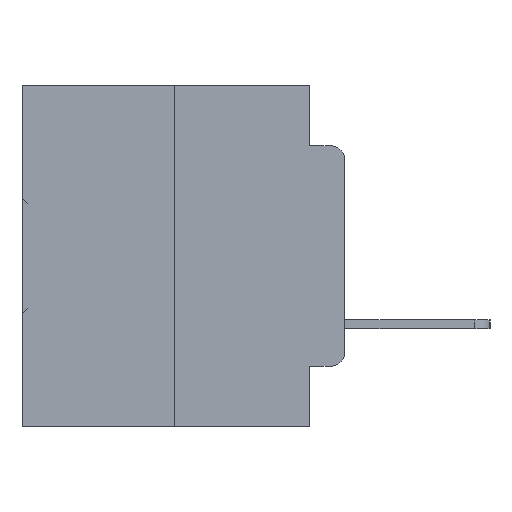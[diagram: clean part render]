
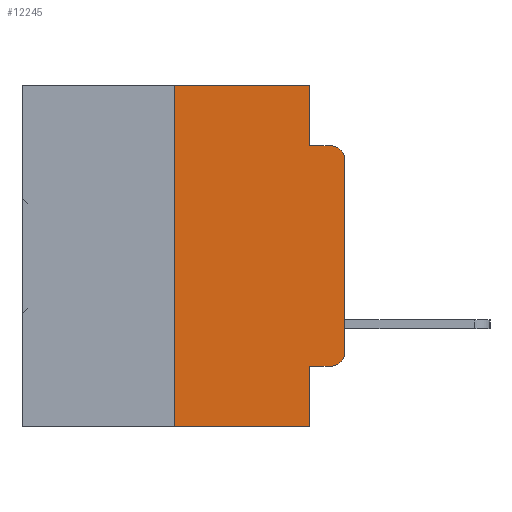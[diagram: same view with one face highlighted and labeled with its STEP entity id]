
A CAD part, left-side view. The second image highlights one B-rep face of the part: STEP entity #12245.
In plain terms, the highlighted planar face has unit normal (-1, 0, 0).
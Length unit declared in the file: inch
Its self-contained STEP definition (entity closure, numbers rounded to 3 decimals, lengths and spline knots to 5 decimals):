
#124 = ORIENTED_EDGE ( 'NONE', *, *, #3405, .T. ) ;
#536 = ORIENTED_EDGE ( 'NONE', *, *, #18207, .F. ) ;
#1031 = CARTESIAN_POINT ( 'NONE',  ( 0., 0.473, -0.5 ) ) ;
#1836 = DIRECTION ( 'NONE',  ( 0., -1., 0. ) ) ;
#2070 = VERTEX_POINT ( 'NONE', #21297 ) ;
#2082 = VERTEX_POINT ( 'NONE', #9404 ) ;
#2098 = CARTESIAN_POINT ( 'NONE',  ( 0., 0.051, -0.0885 ) ) ;
#3405 = EDGE_CURVE ( 'NONE', #30438, #2070, #6796, .T. ) ;
#4148 = DIRECTION ( 'NONE',  ( -1., 0., 0. ) ) ;
#4160 = CARTESIAN_POINT ( 'NONE',  ( 0., 0.051, 0. ) ) ;
#4267 = DIRECTION ( 'NONE',  ( 1., 0., 0. ) ) ;
#4569 = VECTOR ( 'NONE', #27969, 39.37008 ) ;
#4851 = DIRECTION ( 'NONE',  ( 0., -1., 0. ) ) ;
#5417 = LINE ( 'NONE', #4160, #4569 ) ;
#5450 = EDGE_CURVE ( 'NONE', #16482, #11013, #6231, .T. ) ;
#5864 = CARTESIAN_POINT ( 'NONE',  ( 0., 0.25, -0.5 ) ) ;
#5996 = VECTOR ( 'NONE', #30083, 39.37008 ) ;
#6231 = LINE ( 'NONE', #1031, #26460 ) ;
#6551 = DIRECTION ( 'NONE',  ( 0., -1., 0. ) ) ;
#6796 = CIRCLE ( 'NONE', #13078, 0.02 ) ;
#7189 = VERTEX_POINT ( 'NONE', #29967 ) ;
#7971 = EDGE_CURVE ( 'NONE', #2070, #7189, #33920, .T. ) ;
#8220 = CARTESIAN_POINT ( 'NONE',  ( 0., 0.051, -0.5 ) ) ;
#8527 = VECTOR ( 'NONE', #4851, 39.37008 ) ;
#9050 = LINE ( 'NONE', #16271, #15274 ) ;
#9404 = CARTESIAN_POINT ( 'NONE',  ( 0., 0.051, -0.4115 ) ) ;
#9470 = DIRECTION ( 'NONE',  ( -1., 0., 0. ) ) ;
#9798 = EDGE_CURVE ( 'NONE', #7189, #18177, #15871, .T. ) ;
#10254 = VERTEX_POINT ( 'NONE', #13930 ) ;
#11013 = VERTEX_POINT ( 'NONE', #8220 ) ;
#11117 = DIRECTION ( 'NONE',  ( 0., 0., -1. ) ) ;
#12245 = ADVANCED_FACE ( 'NONE', ( #18912 ), #17545, .F. ) ;
#12607 = CARTESIAN_POINT ( 'NONE',  ( 0., 0.051, -0.4115 ) ) ;
#12986 = DIRECTION ( 'NONE',  ( 0., -1., 0. ) ) ;
#13078 = AXIS2_PLACEMENT_3D ( 'NONE', #20061, #4148, #22706 ) ;
#13301 = VECTOR ( 'NONE', #1836, 39.37008 ) ;
#13930 = CARTESIAN_POINT ( 'NONE',  ( 0., 0.25, 0. ) ) ;
#14205 = EDGE_CURVE ( 'NONE', #2082, #30438, #34052, .T. ) ;
#14231 = CARTESIAN_POINT ( 'NONE',  ( 0., 0.051, 0. ) ) ;
#14738 = LINE ( 'NONE', #18208, #20865 ) ;
#14857 = CARTESIAN_POINT ( 'NONE',  ( 0., 0.02, -0.4115 ) ) ;
#15274 = VECTOR ( 'NONE', #11117, 39.37008 ) ;
#15871 = CIRCLE ( 'NONE', #29210, 0.02 ) ;
#15982 = EDGE_CURVE ( 'NONE', #2082, #11013, #9050, .T. ) ;
#16271 = CARTESIAN_POINT ( 'NONE',  ( 0., 0.051, 0. ) ) ;
#16482 = VERTEX_POINT ( 'NONE', #5864 ) ;
#17545 = PLANE ( 'NONE',  #25097 ) ;
#18161 = EDGE_CURVE ( 'NONE', #31803, #18177, #29434, .T. ) ;
#18177 = VERTEX_POINT ( 'NONE', #20736 ) ;
#18207 = EDGE_CURVE ( 'NONE', #10254, #21811, #14738, .T. ) ;
#18208 = CARTESIAN_POINT ( 'NONE',  ( 0., 0.473, 0. ) ) ;
#18912 = FACE_OUTER_BOUND ( 'NONE', #21444, .T. ) ;
#19676 = VECTOR ( 'NONE', #30300, 39.37008 ) ;
#20061 = CARTESIAN_POINT ( 'NONE',  ( 0., 0.02, -0.3915 ) ) ;
#20204 = ORIENTED_EDGE ( 'NONE', *, *, #18161, .F. ) ;
#20512 = LINE ( 'NONE', #22442, #19676 ) ;
#20582 = EDGE_CURVE ( 'NONE', #21811, #31803, #5417, .T. ) ;
#20736 = CARTESIAN_POINT ( 'NONE',  ( 0., 0.02, -0.0885 ) ) ;
#20865 = VECTOR ( 'NONE', #12986, 39.37008 ) ;
#21297 = CARTESIAN_POINT ( 'NONE',  ( 0., 0., -0.3915 ) ) ;
#21444 = EDGE_LOOP ( 'NONE', ( #31603, #32397, #20204, #34029, #536, #29586, #23498, #25140, #33646, #124 ) ) ;
#21642 = CARTESIAN_POINT ( 'NONE',  ( 0., 0.051, -0.0885 ) ) ;
#21811 = VERTEX_POINT ( 'NONE', #14231 ) ;
#22235 = CARTESIAN_POINT ( 'NONE',  ( 0., 0., 0. ) ) ;
#22442 = CARTESIAN_POINT ( 'NONE',  ( 0., 0.25, 0. ) ) ;
#22706 = DIRECTION ( 'NONE',  ( 0., 0., -1. ) ) ;
#22707 = CARTESIAN_POINT ( 'NONE',  ( 0., 0.473, 0. ) ) ;
#22818 = DIRECTION ( 'NONE',  ( 0., 0., -1. ) ) ;
#23498 = ORIENTED_EDGE ( 'NONE', *, *, #5450, .T. ) ;
#25097 = AXIS2_PLACEMENT_3D ( 'NONE', #22707, #4267, #22818 ) ;
#25140 = ORIENTED_EDGE ( 'NONE', *, *, #15982, .F. ) ;
#25181 = CARTESIAN_POINT ( 'NONE',  ( 0., 0.02, -0.1085 ) ) ;
#26460 = VECTOR ( 'NONE', #6551, 39.37008 ) ;
#27777 = DIRECTION ( 'NONE',  ( 0., 0., -1. ) ) ;
#27969 = DIRECTION ( 'NONE',  ( 0., 0., -1. ) ) ;
#28241 = EDGE_CURVE ( 'NONE', #16482, #10254, #20512, .T. ) ;
#29210 = AXIS2_PLACEMENT_3D ( 'NONE', #25181, #9470, #27777 ) ;
#29434 = LINE ( 'NONE', #2098, #8527 ) ;
#29586 = ORIENTED_EDGE ( 'NONE', *, *, #28241, .F. ) ;
#29967 = CARTESIAN_POINT ( 'NONE',  ( 0., 0., -0.1085 ) ) ;
#30083 = DIRECTION ( 'NONE',  ( 0., 0., 1. ) ) ;
#30300 = DIRECTION ( 'NONE',  ( 0., 0., 1. ) ) ;
#30438 = VERTEX_POINT ( 'NONE', #14857 ) ;
#31603 = ORIENTED_EDGE ( 'NONE', *, *, #7971, .T. ) ;
#31803 = VERTEX_POINT ( 'NONE', #21642 ) ;
#32397 = ORIENTED_EDGE ( 'NONE', *, *, #9798, .T. ) ;
#33646 = ORIENTED_EDGE ( 'NONE', *, *, #14205, .T. ) ;
#33920 = LINE ( 'NONE', #22235, #5996 ) ;
#34029 = ORIENTED_EDGE ( 'NONE', *, *, #20582, .F. ) ;
#34052 = LINE ( 'NONE', #12607, #13301 ) ;
